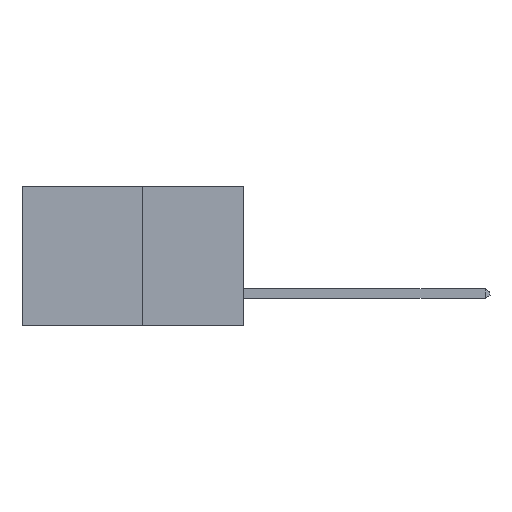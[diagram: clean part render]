
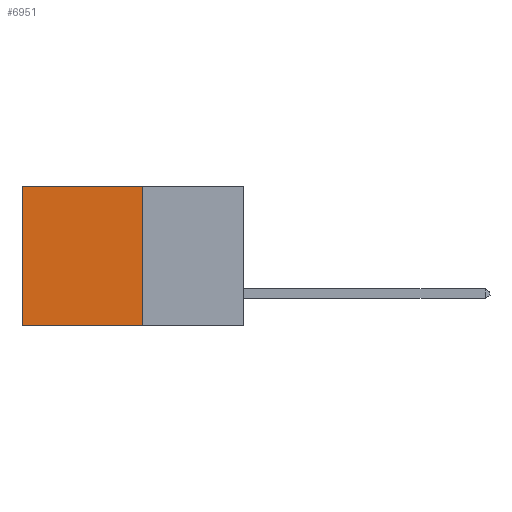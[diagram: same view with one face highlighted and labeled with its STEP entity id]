
A CAD part, left-side view. The second image highlights one B-rep face of the part: STEP entity #6951.
In plain terms, the highlighted planar face has unit normal (-1, 0, 0).
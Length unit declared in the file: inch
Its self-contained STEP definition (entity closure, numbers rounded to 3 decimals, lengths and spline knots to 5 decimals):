
#51 = DIRECTION ( 'NONE',  ( 0., 1., 0. ) ) ;
#166 = ORIENTED_EDGE ( 'NONE', *, *, #3149, .T. ) ;
#376 = CARTESIAN_POINT ( 'NONE',  ( 0.277, 0.27, -0.37 ) ) ;
#925 = CARTESIAN_POINT ( 'NONE',  ( 0.277, 0.27, 0. ) ) ;
#1095 = LINE ( 'NONE', #376, #7114 ) ;
#1262 = CARTESIAN_POINT ( 'NONE',  ( 0.277, 0.27, -0.37 ) ) ;
#1781 = DIRECTION ( 'NONE',  ( 1., 0., 0. ) ) ;
#2101 = CARTESIAN_POINT ( 'NONE',  ( 0.277, 0.59, -0.37 ) ) ;
#2422 = DIRECTION ( 'NONE',  ( 0., 1., 0. ) ) ;
#2435 = PLANE ( 'NONE',  #9716 ) ;
#2439 = ORIENTED_EDGE ( 'NONE', *, *, #7024, .T. ) ;
#3143 = VECTOR ( 'NONE', #5343, 39.37008 ) ;
#3149 = EDGE_CURVE ( 'NONE', #4633, #4912, #6959, .T. ) ;
#3290 = VERTEX_POINT ( 'NONE', #5066 ) ;
#3481 = VERTEX_POINT ( 'NONE', #4898 ) ;
#4063 = CARTESIAN_POINT ( 'NONE',  ( 0.277, 0.59, -0.37 ) ) ;
#4601 = EDGE_CURVE ( 'NONE', #3290, #3481, #9548, .T. ) ;
#4633 = VERTEX_POINT ( 'NONE', #4738 ) ;
#4738 = CARTESIAN_POINT ( 'NONE',  ( 0.277, 0.59, 0. ) ) ;
#4898 = CARTESIAN_POINT ( 'NONE',  ( 0.277, 0.27, -0.37 ) ) ;
#4912 = VERTEX_POINT ( 'NONE', #4063 ) ;
#5066 = CARTESIAN_POINT ( 'NONE',  ( 0.277, 0.27, 0. ) ) ;
#5343 = DIRECTION ( 'NONE',  ( 0., 0., -1. ) ) ;
#5572 = EDGE_CURVE ( 'NONE', #3481, #4912, #1095, .T. ) ;
#5896 = CARTESIAN_POINT ( 'NONE',  ( 0.277, 0.27, -0.37 ) ) ;
#6619 = LINE ( 'NONE', #925, #8130 ) ;
#6951 = ADVANCED_FACE ( 'NONE', ( #7549 ), #2435, .F. ) ;
#6959 = LINE ( 'NONE', #2101, #3143 ) ;
#7024 = EDGE_CURVE ( 'NONE', #3290, #4633, #6619, .T. ) ;
#7114 = VECTOR ( 'NONE', #2422, 39.37008 ) ;
#7345 = EDGE_LOOP ( 'NONE', ( #166, #7707, #8173, #2439 ) ) ;
#7549 = FACE_OUTER_BOUND ( 'NONE', #7345, .T. ) ;
#7616 = VECTOR ( 'NONE', #8191, 39.37008 ) ;
#7707 = ORIENTED_EDGE ( 'NONE', *, *, #5572, .F. ) ;
#7720 = DIRECTION ( 'NONE',  ( 0., 0., -1. ) ) ;
#8130 = VECTOR ( 'NONE', #51, 39.37008 ) ;
#8173 = ORIENTED_EDGE ( 'NONE', *, *, #4601, .F. ) ;
#8191 = DIRECTION ( 'NONE',  ( 0., 0., -1. ) ) ;
#9548 = LINE ( 'NONE', #1262, #7616 ) ;
#9716 = AXIS2_PLACEMENT_3D ( 'NONE', #5896, #1781, #7720 ) ;
